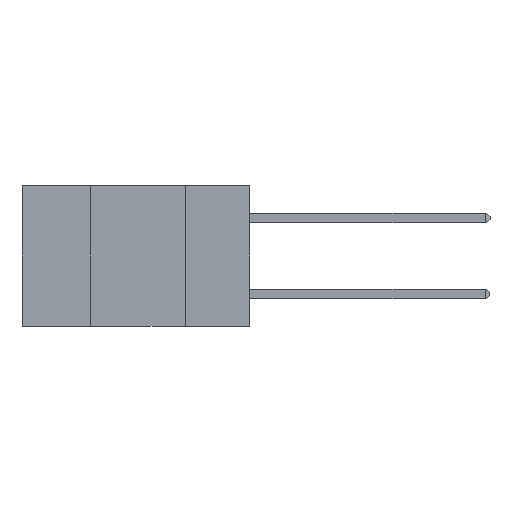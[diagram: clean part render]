
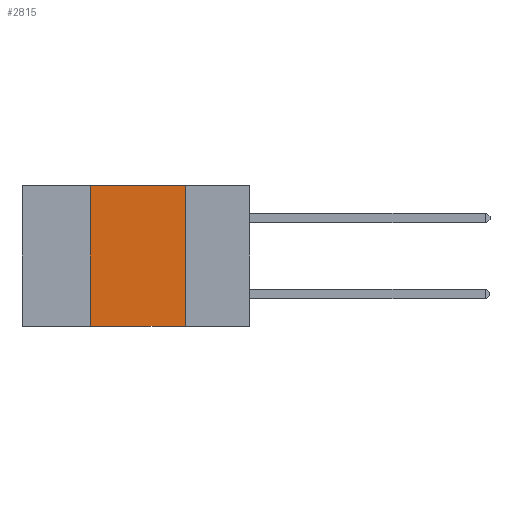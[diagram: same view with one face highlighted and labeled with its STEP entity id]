
A CAD part, left-side view. The second image highlights one B-rep face of the part: STEP entity #2815.
In plain terms, the highlighted planar face has unit normal (-1, 0, 0).
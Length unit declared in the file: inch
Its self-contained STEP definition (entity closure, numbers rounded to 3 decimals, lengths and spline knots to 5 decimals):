
#131 = DIRECTION ( 'NONE',  ( 0., 0., -1. ) ) ;
#691 = AXIS2_PLACEMENT_3D ( 'NONE', #3701, #3399, #3206 ) ;
#1698 = VERTEX_POINT ( 'NONE', #15027 ) ;
#1914 = VECTOR ( 'NONE', #131, 39.37008 ) ;
#2815 = ADVANCED_FACE ( 'NONE', ( #8026 ), #3500, .F. ) ;
#3056 = LINE ( 'NONE', #13047, #15234 ) ;
#3206 = DIRECTION ( 'NONE',  ( 0., 0., -1. ) ) ;
#3321 = VECTOR ( 'NONE', #13584, 39.37008 ) ;
#3399 = DIRECTION ( 'NONE',  ( 1., 0., 0. ) ) ;
#3500 = PLANE ( 'NONE',  #691 ) ;
#3701 = CARTESIAN_POINT ( 'NONE',  ( 0., 0.6, 0. ) ) ;
#3863 = EDGE_CURVE ( 'NONE', #1698, #14046, #7736, .T. ) ;
#4009 = VERTEX_POINT ( 'NONE', #9295 ) ;
#7324 = VERTEX_POINT ( 'NONE', #9404 ) ;
#7481 = ORIENTED_EDGE ( 'NONE', *, *, #10511, .F. ) ;
#7736 = LINE ( 'NONE', #13916, #13171 ) ;
#7869 = EDGE_CURVE ( 'NONE', #7324, #4009, #9972, .T. ) ;
#8026 = FACE_OUTER_BOUND ( 'NONE', #11907, .T. ) ;
#8247 = CARTESIAN_POINT ( 'NONE',  ( 0., 0.17, -0.37 ) ) ;
#8589 = LINE ( 'NONE', #14633, #1914 ) ;
#9295 = CARTESIAN_POINT ( 'NONE',  ( 0., 0.17, 0. ) ) ;
#9404 = CARTESIAN_POINT ( 'NONE',  ( 0., 0.42, 0. ) ) ;
#9447 = EDGE_CURVE ( 'NONE', #4009, #14046, #8589, .T. ) ;
#9736 = DIRECTION ( 'NONE',  ( 0., 0., 1. ) ) ;
#9972 = LINE ( 'NONE', #12462, #3321 ) ;
#10034 = ORIENTED_EDGE ( 'NONE', *, *, #7869, .F. ) ;
#10511 = EDGE_CURVE ( 'NONE', #1698, #7324, #3056, .T. ) ;
#11907 = EDGE_LOOP ( 'NONE', ( #12265, #10034, #7481, #13655 ) ) ;
#12265 = ORIENTED_EDGE ( 'NONE', *, *, #9447, .F. ) ;
#12462 = CARTESIAN_POINT ( 'NONE',  ( 0., 0.6, 0. ) ) ;
#13047 = CARTESIAN_POINT ( 'NONE',  ( 0., 0.42, 0. ) ) ;
#13171 = VECTOR ( 'NONE', #13782, 39.37008 ) ;
#13584 = DIRECTION ( 'NONE',  ( 0., -1., 0. ) ) ;
#13655 = ORIENTED_EDGE ( 'NONE', *, *, #3863, .T. ) ;
#13782 = DIRECTION ( 'NONE',  ( 0., -1., 0. ) ) ;
#13916 = CARTESIAN_POINT ( 'NONE',  ( 0., 0.6, -0.37 ) ) ;
#14046 = VERTEX_POINT ( 'NONE', #8247 ) ;
#14633 = CARTESIAN_POINT ( 'NONE',  ( 0., 0.17, 0. ) ) ;
#15027 = CARTESIAN_POINT ( 'NONE',  ( 0., 0.42, -0.37 ) ) ;
#15234 = VECTOR ( 'NONE', #9736, 39.37008 ) ;
